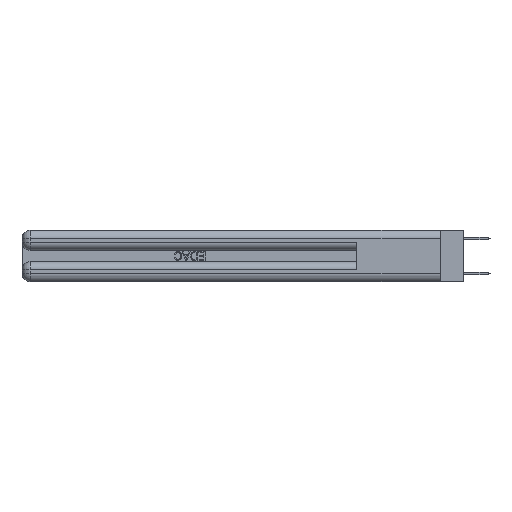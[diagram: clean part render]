
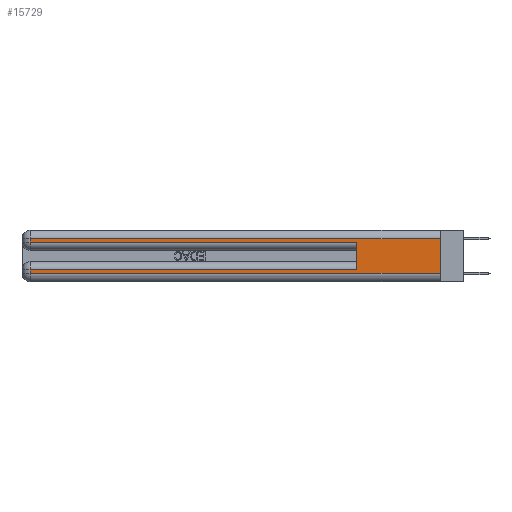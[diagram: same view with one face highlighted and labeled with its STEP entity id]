
A CAD part, left-side view. The second image highlights one B-rep face of the part: STEP entity #15729.
In plain terms, the highlighted planar face has unit normal (-1, 0, 0).
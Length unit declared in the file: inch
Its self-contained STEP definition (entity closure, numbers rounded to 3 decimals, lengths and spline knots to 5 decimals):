
#590 = VERTEX_POINT ( 'NONE', #23407 ) ;
#800 = CARTESIAN_POINT ( 'NONE',  ( 0., 0., 0.06 ) ) ;
#970 = VECTOR ( 'NONE', #22363, 39.37008 ) ;
#1529 = AXIS2_PLACEMENT_3D ( 'NONE', #2729, #28864, #26986 ) ;
#1561 = VERTEX_POINT ( 'NONE', #26428 ) ;
#1632 = DIRECTION ( 'NONE',  ( 0., 1., 0. ) ) ;
#2268 = EDGE_CURVE ( 'NONE', #22526, #1561, #8650, .T. ) ;
#2395 = CARTESIAN_POINT ( 'NONE',  ( 0., 2.94, 0.06 ) ) ;
#2724 = VECTOR ( 'NONE', #3978, 39.37008 ) ;
#2729 = CARTESIAN_POINT ( 'NONE',  ( 0., 0., 0.37 ) ) ;
#3442 = DIRECTION ( 'NONE',  ( 0., 0., -1. ) ) ;
#3978 = DIRECTION ( 'NONE',  ( 0., 1., 0. ) ) ;
#3993 = CARTESIAN_POINT ( 'NONE',  ( 0., 0., 0.06 ) ) ;
#4384 = CARTESIAN_POINT ( 'NONE',  ( 0., 2.94, 0.285 ) ) ;
#4995 = DIRECTION ( 'NONE',  ( 0., -1., 0. ) ) ;
#5418 = DIRECTION ( 'NONE',  ( 0., 0., -1. ) ) ;
#5891 = EDGE_CURVE ( 'NONE', #20143, #20818, #16131, .T. ) ;
#6060 = ORIENTED_EDGE ( 'NONE', *, *, #18522, .T. ) ;
#6134 = ORIENTED_EDGE ( 'NONE', *, *, #13170, .F. ) ;
#6966 = ORIENTED_EDGE ( 'NONE', *, *, #15294, .F. ) ;
#8050 = LINE ( 'NONE', #14747, #970 ) ;
#8407 = LINE ( 'NONE', #20397, #18301 ) ;
#8650 = LINE ( 'NONE', #27621, #2724 ) ;
#8818 = DIRECTION ( 'NONE',  ( 0., -1., 0. ) ) ;
#10567 = CARTESIAN_POINT ( 'NONE',  ( 0., 2.94, 0.37 ) ) ;
#10601 = EDGE_CURVE ( 'NONE', #1561, #29044, #26592, .T. ) ;
#11100 = VECTOR ( 'NONE', #8818, 39.37008 ) ;
#11368 = ORIENTED_EDGE ( 'NONE', *, *, #5891, .T. ) ;
#12919 = DIRECTION ( 'NONE',  ( 0., 0., -1. ) ) ;
#13170 = EDGE_CURVE ( 'NONE', #22526, #20818, #14607, .T. ) ;
#13373 = VECTOR ( 'NONE', #12919, 39.37008 ) ;
#14499 = CARTESIAN_POINT ( 'NONE',  ( 0., 0., 0.285 ) ) ;
#14607 = LINE ( 'NONE', #17080, #29655 ) ;
#14747 = CARTESIAN_POINT ( 'NONE',  ( 0., 0.6, 0.145 ) ) ;
#14913 = EDGE_LOOP ( 'NONE', ( #6134, #23536, #21056, #23373, #6966, #6060, #29687, #11368 ) ) ;
#15106 = CARTESIAN_POINT ( 'NONE',  ( 0., 0.6, 0.285 ) ) ;
#15294 = EDGE_CURVE ( 'NONE', #590, #19529, #8050, .T. ) ;
#15729 = ADVANCED_FACE ( 'NONE', ( #26366 ), #29015, .F. ) ;
#16131 = LINE ( 'NONE', #3993, #11100 ) ;
#16812 = LINE ( 'NONE', #14499, #19310 ) ;
#17080 = CARTESIAN_POINT ( 'NONE',  ( 0., 0., 0.37 ) ) ;
#17504 = VECTOR ( 'NONE', #1632, 39.37008 ) ;
#17753 = VERTEX_POINT ( 'NONE', #25989 ) ;
#18301 = VECTOR ( 'NONE', #3442, 39.37008 ) ;
#18522 = EDGE_CURVE ( 'NONE', #590, #17753, #25126, .T. ) ;
#19310 = VECTOR ( 'NONE', #4995, 39.37008 ) ;
#19529 = VERTEX_POINT ( 'NONE', #15106 ) ;
#20143 = VERTEX_POINT ( 'NONE', #2395 ) ;
#20397 = CARTESIAN_POINT ( 'NONE',  ( 0., 2.94, 0.37 ) ) ;
#20625 = CARTESIAN_POINT ( 'NONE',  ( 0., 0., 0.085 ) ) ;
#20818 = VERTEX_POINT ( 'NONE', #800 ) ;
#21056 = ORIENTED_EDGE ( 'NONE', *, *, #10601, .T. ) ;
#22363 = DIRECTION ( 'NONE',  ( 0., 0., 1. ) ) ;
#22526 = VERTEX_POINT ( 'NONE', #27503 ) ;
#23373 = ORIENTED_EDGE ( 'NONE', *, *, #27902, .T. ) ;
#23407 = CARTESIAN_POINT ( 'NONE',  ( 0., 0.6, 0.085 ) ) ;
#23536 = ORIENTED_EDGE ( 'NONE', *, *, #2268, .T. ) ;
#25126 = LINE ( 'NONE', #20625, #17504 ) ;
#25989 = CARTESIAN_POINT ( 'NONE',  ( 0., 2.94, 0.085 ) ) ;
#26366 = FACE_OUTER_BOUND ( 'NONE', #14913, .T. ) ;
#26428 = CARTESIAN_POINT ( 'NONE',  ( 0., 2.94, 0.31 ) ) ;
#26592 = LINE ( 'NONE', #10567, #13373 ) ;
#26986 = DIRECTION ( 'NONE',  ( 0., 0., -1. ) ) ;
#27503 = CARTESIAN_POINT ( 'NONE',  ( 0., 0., 0.31 ) ) ;
#27621 = CARTESIAN_POINT ( 'NONE',  ( 0., 0., 0.31 ) ) ;
#27902 = EDGE_CURVE ( 'NONE', #29044, #19529, #16812, .T. ) ;
#28864 = DIRECTION ( 'NONE',  ( 1., 0., 0. ) ) ;
#29015 = PLANE ( 'NONE',  #1529 ) ;
#29044 = VERTEX_POINT ( 'NONE', #4384 ) ;
#29252 = EDGE_CURVE ( 'NONE', #17753, #20143, #8407, .T. ) ;
#29655 = VECTOR ( 'NONE', #5418, 39.37008 ) ;
#29687 = ORIENTED_EDGE ( 'NONE', *, *, #29252, .T. ) ;
